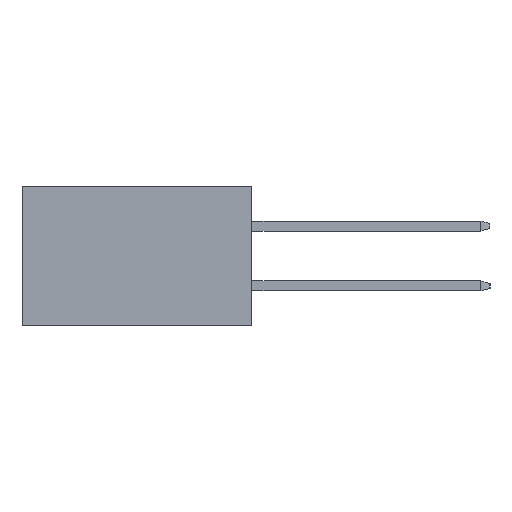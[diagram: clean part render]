
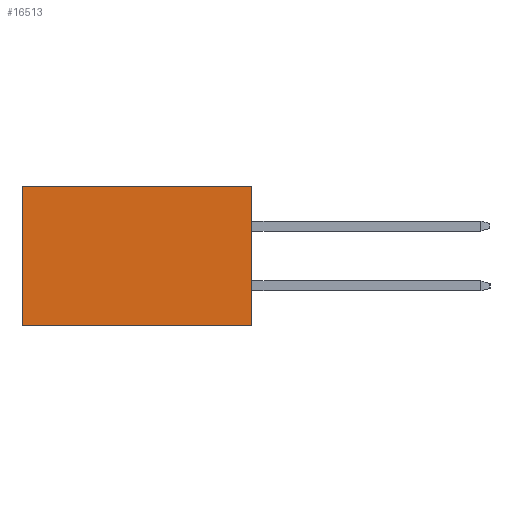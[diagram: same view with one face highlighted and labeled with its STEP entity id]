
A CAD part, left-side view. The second image highlights one B-rep face of the part: STEP entity #16513.
In plain terms, the highlighted planar face has unit normal (-1, 0, 0).
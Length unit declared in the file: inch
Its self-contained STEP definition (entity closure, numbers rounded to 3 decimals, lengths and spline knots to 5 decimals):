
#286 = EDGE_CURVE ( 'NONE', #8993, #14991, #7226, .T. ) ;
#451 = EDGE_LOOP ( 'NONE', ( #5420, #1242, #8176, #20699 ) ) ;
#512 = CARTESIAN_POINT ( 'NONE',  ( 0.3205, 0., -0.437 ) ) ;
#1132 = CARTESIAN_POINT ( 'NONE',  ( 0.3205, 0.72, 0. ) ) ;
#1242 = ORIENTED_EDGE ( 'NONE', *, *, #3718, .F. ) ;
#3273 = LINE ( 'NONE', #19473, #17198 ) ;
#3509 = VECTOR ( 'NONE', #13766, 39.37008 ) ;
#3718 = EDGE_CURVE ( 'NONE', #14991, #6196, #3273, .T. ) ;
#4439 = EDGE_CURVE ( 'NONE', #9197, #6196, #9185, .T. ) ;
#4510 = CARTESIAN_POINT ( 'NONE',  ( 0.3205, 0., -0.437 ) ) ;
#5332 = AXIS2_PLACEMENT_3D ( 'NONE', #4510, #12518, #5809 ) ;
#5420 = ORIENTED_EDGE ( 'NONE', *, *, #4439, .T. ) ;
#5809 = DIRECTION ( 'NONE',  ( 0., 0., -1. ) ) ;
#6196 = VERTEX_POINT ( 'NONE', #11792 ) ;
#7122 = DIRECTION ( 'NONE',  ( 0., 1., 0. ) ) ;
#7226 = LINE ( 'NONE', #512, #8415 ) ;
#8176 = ORIENTED_EDGE ( 'NONE', *, *, #286, .F. ) ;
#8415 = VECTOR ( 'NONE', #20225, 39.37008 ) ;
#8416 = VECTOR ( 'NONE', #7122, 39.37008 ) ;
#8993 = VERTEX_POINT ( 'NONE', #16615 ) ;
#9185 = LINE ( 'NONE', #15372, #3509 ) ;
#9197 = VERTEX_POINT ( 'NONE', #1132 ) ;
#9976 = DIRECTION ( 'NONE',  ( 0., 1., 0. ) ) ;
#11792 = CARTESIAN_POINT ( 'NONE',  ( 0.3205, 0.72, -0.437 ) ) ;
#12409 = LINE ( 'NONE', #16802, #8416 ) ;
#12518 = DIRECTION ( 'NONE',  ( 1., 0., 0. ) ) ;
#12946 = CARTESIAN_POINT ( 'NONE',  ( 0.3205, 0., -0.437 ) ) ;
#13766 = DIRECTION ( 'NONE',  ( 0., 0., -1. ) ) ;
#14991 = VERTEX_POINT ( 'NONE', #12946 ) ;
#15372 = CARTESIAN_POINT ( 'NONE',  ( 0.3205, 0.72, -0.437 ) ) ;
#16513 = ADVANCED_FACE ( 'NONE', ( #20621 ), #17312, .F. ) ;
#16615 = CARTESIAN_POINT ( 'NONE',  ( 0.3205, 0., 0. ) ) ;
#16802 = CARTESIAN_POINT ( 'NONE',  ( 0.3205, 0., 0. ) ) ;
#17198 = VECTOR ( 'NONE', #9976, 39.37008 ) ;
#17312 = PLANE ( 'NONE',  #5332 ) ;
#18517 = EDGE_CURVE ( 'NONE', #8993, #9197, #12409, .T. ) ;
#19473 = CARTESIAN_POINT ( 'NONE',  ( 0.3205, 0., -0.437 ) ) ;
#20225 = DIRECTION ( 'NONE',  ( 0., 0., -1. ) ) ;
#20621 = FACE_OUTER_BOUND ( 'NONE', #451, .T. ) ;
#20699 = ORIENTED_EDGE ( 'NONE', *, *, #18517, .T. ) ;
